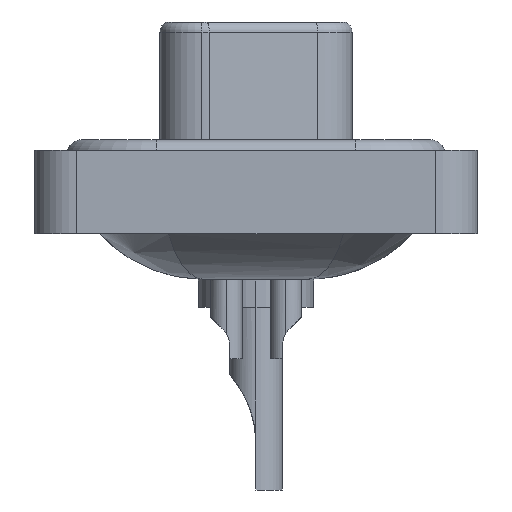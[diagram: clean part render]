
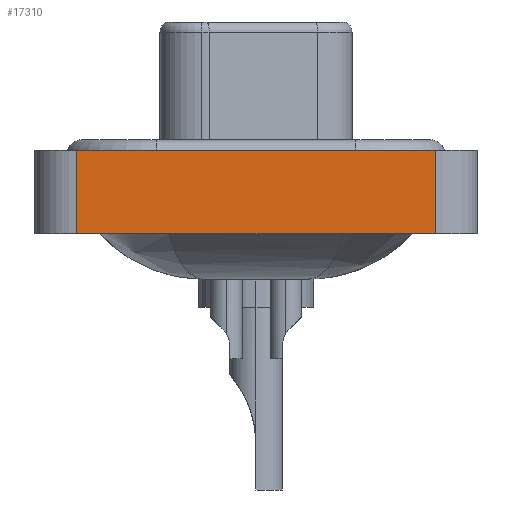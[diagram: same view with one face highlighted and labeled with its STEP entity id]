
A CAD part, left-side view. The second image highlights one B-rep face of the part: STEP entity #17310.
In plain terms, the highlighted planar face has unit normal (-1, 0, 0).
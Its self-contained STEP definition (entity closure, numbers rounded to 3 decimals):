
#36 = EDGE_CURVE ( 'NONE', #4232, #13957, #8204, .T. ) ;
#53 = VERTEX_POINT ( 'NONE', #18870 ) ;
#2098 = LINE ( 'NONE', #16509, #7157 ) ;
#3724 = AXIS2_PLACEMENT_3D ( 'NONE', #7802, #17799, #16098 ) ;
#4232 = VERTEX_POINT ( 'NONE', #4286 ) ;
#4286 = CARTESIAN_POINT ( 'NONE',  ( -7.3, -8.55, -3.6 ) ) ;
#5043 = CARTESIAN_POINT ( 'NONE',  ( -7.3, -8.55, 0.4 ) ) ;
#6927 = DIRECTION ( 'NONE',  ( 0., -1., 0. ) ) ;
#7157 = VECTOR ( 'NONE', #6927, 1000. ) ;
#7433 = VERTEX_POINT ( 'NONE', #9548 ) ;
#7802 = CARTESIAN_POINT ( 'NONE',  ( -7.3, -8.55, -3.6 ) ) ;
#8204 = LINE ( 'NONE', #14781, #8623 ) ;
#8618 = VECTOR ( 'NONE', #18339, 1000. ) ;
#8623 = VECTOR ( 'NONE', #13167, 1000. ) ;
#8671 = CARTESIAN_POINT ( 'NONE',  ( -7.3, 8.55, -3.6 ) ) ;
#9548 = CARTESIAN_POINT ( 'NONE',  ( -7.3, 8.55, -3.6 ) ) ;
#9628 = PLANE ( 'NONE',  #3724 ) ;
#10065 = ORIENTED_EDGE ( 'NONE', *, *, #17067, .F. ) ;
#10276 = CARTESIAN_POINT ( 'NONE',  ( -7.3, -8.55, -3.6 ) ) ;
#11023 = ORIENTED_EDGE ( 'NONE', *, *, #36, .T. ) ;
#13167 = DIRECTION ( 'NONE',  ( 0., 0., 1. ) ) ;
#13284 = LINE ( 'NONE', #10276, #8618 ) ;
#13477 = VECTOR ( 'NONE', #15254, 1000. ) ;
#13746 = ORIENTED_EDGE ( 'NONE', *, *, #14134, .T. ) ;
#13957 = VERTEX_POINT ( 'NONE', #5043 ) ;
#14134 = EDGE_CURVE ( 'NONE', #7433, #4232, #13284, .T. ) ;
#14672 = FACE_OUTER_BOUND ( 'NONE', #18911, .T. ) ;
#14781 = CARTESIAN_POINT ( 'NONE',  ( -7.3, -8.55, -3.6 ) ) ;
#15254 = DIRECTION ( 'NONE',  ( 0., 0., 1. ) ) ;
#15932 = ORIENTED_EDGE ( 'NONE', *, *, #19601, .F. ) ;
#16098 = DIRECTION ( 'NONE',  ( 0., 0., 1. ) ) ;
#16509 = CARTESIAN_POINT ( 'NONE',  ( -7.3, -8.55, 0.4 ) ) ;
#16959 = LINE ( 'NONE', #8671, #13477 ) ;
#17067 = EDGE_CURVE ( 'NONE', #7433, #53, #16959, .T. ) ;
#17310 = ADVANCED_FACE ( 'NONE', ( #14672 ), #9628, .T. ) ;
#17799 = DIRECTION ( 'NONE',  ( -1., 0., 0. ) ) ;
#18339 = DIRECTION ( 'NONE',  ( 0., -1., 0. ) ) ;
#18870 = CARTESIAN_POINT ( 'NONE',  ( -7.3, 8.55, 0.4 ) ) ;
#18911 = EDGE_LOOP ( 'NONE', ( #11023, #15932, #10065, #13746 ) ) ;
#19601 = EDGE_CURVE ( 'NONE', #53, #13957, #2098, .T. ) ;
